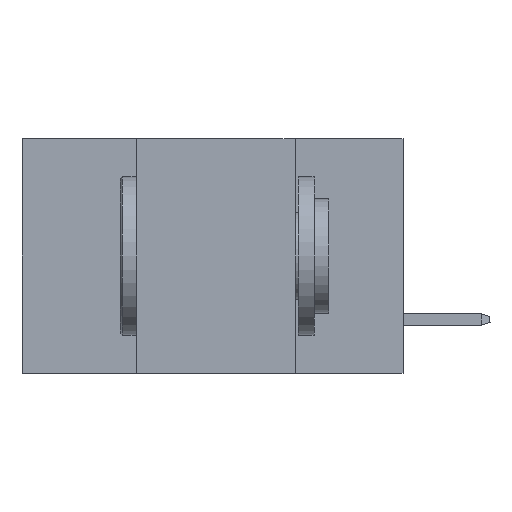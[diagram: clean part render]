
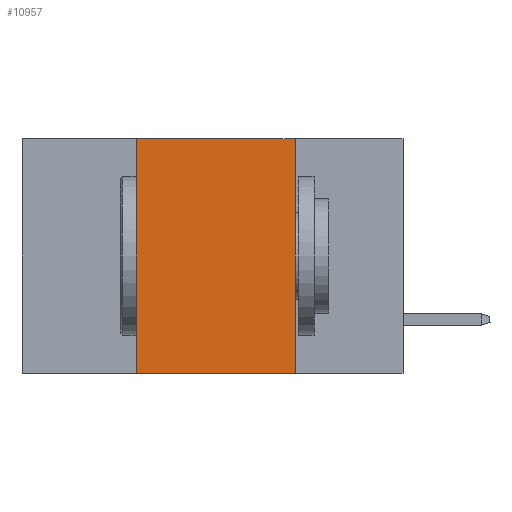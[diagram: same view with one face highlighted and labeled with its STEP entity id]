
A CAD part, left-side view. The second image highlights one B-rep face of the part: STEP entity #10957.
In plain terms, the highlighted planar face has unit normal (-1, 0, 0).
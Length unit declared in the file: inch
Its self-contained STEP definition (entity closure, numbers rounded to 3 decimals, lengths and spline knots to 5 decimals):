
#457 = VECTOR ( 'NONE', #2100, 39.37008 ) ;
#775 = EDGE_LOOP ( 'NONE', ( #11501, #19099, #3060, #12314 ) ) ;
#1140 = EDGE_CURVE ( 'NONE', #8898, #16326, #4509, .T. ) ;
#1263 = CARTESIAN_POINT ( 'NONE',  ( 0., 0.6, -0.37 ) ) ;
#2100 = DIRECTION ( 'NONE',  ( 0., -1., 0. ) ) ;
#2226 = CARTESIAN_POINT ( 'NONE',  ( 0., 0.42, -0.37 ) ) ;
#2596 = DIRECTION ( 'NONE',  ( 0., 0., -1. ) ) ;
#3060 = ORIENTED_EDGE ( 'NONE', *, *, #16321, .F. ) ;
#4509 = LINE ( 'NONE', #1263, #7108 ) ;
#4983 = VERTEX_POINT ( 'NONE', #14298 ) ;
#5217 = PLANE ( 'NONE',  #14846 ) ;
#5420 = CARTESIAN_POINT ( 'NONE',  ( 0., 0.6, 0. ) ) ;
#7037 = DIRECTION ( 'NONE',  ( 0., 0., -1. ) ) ;
#7108 = VECTOR ( 'NONE', #9262, 39.37008 ) ;
#8898 = VERTEX_POINT ( 'NONE', #2226 ) ;
#9262 = DIRECTION ( 'NONE',  ( 0., -1., 0. ) ) ;
#9627 = CARTESIAN_POINT ( 'NONE',  ( 0., 0.42, 0. ) ) ;
#9957 = LINE ( 'NONE', #18285, #17706 ) ;
#10437 = VERTEX_POINT ( 'NONE', #20032 ) ;
#10801 = DIRECTION ( 'NONE',  ( 1., 0., 0. ) ) ;
#10957 = ADVANCED_FACE ( 'NONE', ( #13430 ), #5217, .F. ) ;
#11501 = ORIENTED_EDGE ( 'NONE', *, *, #19347, .F. ) ;
#12314 = ORIENTED_EDGE ( 'NONE', *, *, #1140, .T. ) ;
#12452 = VECTOR ( 'NONE', #14499, 39.37008 ) ;
#13430 = FACE_OUTER_BOUND ( 'NONE', #775, .T. ) ;
#14298 = CARTESIAN_POINT ( 'NONE',  ( 0., 0.42, 0. ) ) ;
#14499 = DIRECTION ( 'NONE',  ( 0., 0., 1. ) ) ;
#14846 = AXIS2_PLACEMENT_3D ( 'NONE', #5420, #10801, #2596 ) ;
#16321 = EDGE_CURVE ( 'NONE', #8898, #4983, #17951, .T. ) ;
#16326 = VERTEX_POINT ( 'NONE', #19131 ) ;
#17706 = VECTOR ( 'NONE', #7037, 39.37008 ) ;
#17951 = LINE ( 'NONE', #9627, #12452 ) ;
#18285 = CARTESIAN_POINT ( 'NONE',  ( 0., 0.17, 0. ) ) ;
#18822 = CARTESIAN_POINT ( 'NONE',  ( 0., 0.6, 0. ) ) ;
#18981 = EDGE_CURVE ( 'NONE', #4983, #10437, #20130, .T. ) ;
#19099 = ORIENTED_EDGE ( 'NONE', *, *, #18981, .F. ) ;
#19131 = CARTESIAN_POINT ( 'NONE',  ( 0., 0.17, -0.37 ) ) ;
#19347 = EDGE_CURVE ( 'NONE', #10437, #16326, #9957, .T. ) ;
#20032 = CARTESIAN_POINT ( 'NONE',  ( 0., 0.17, 0. ) ) ;
#20130 = LINE ( 'NONE', #18822, #457 ) ;
